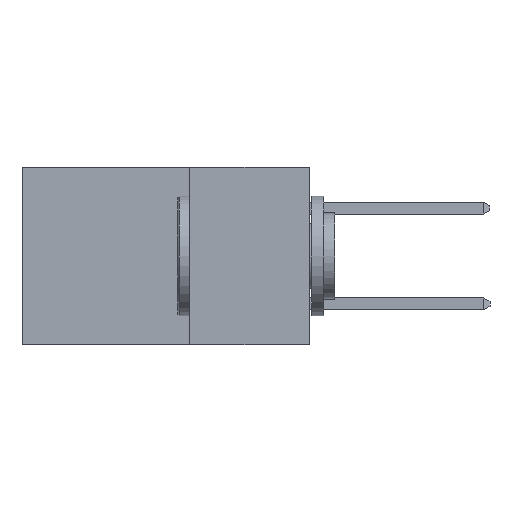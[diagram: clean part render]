
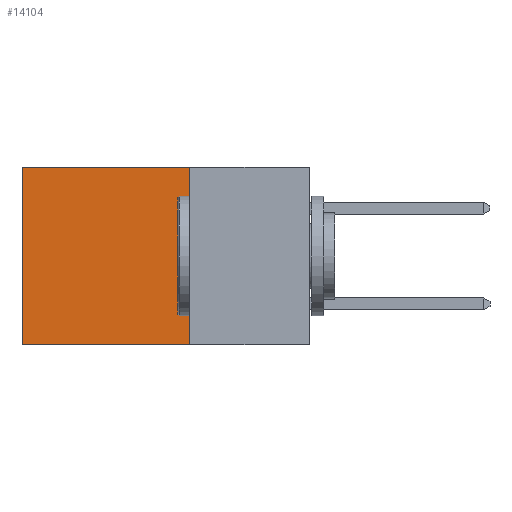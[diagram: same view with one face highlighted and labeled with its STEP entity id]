
A CAD part, left-side view. The second image highlights one B-rep face of the part: STEP entity #14104.
In plain terms, the highlighted planar face has unit normal (-1, 0, 0).
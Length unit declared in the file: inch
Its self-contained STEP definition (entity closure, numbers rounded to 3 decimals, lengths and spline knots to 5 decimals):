
#1216 = DIRECTION ( 'NONE',  ( 0., 0., -1. ) ) ;
#1329 = VERTEX_POINT ( 'NONE', #12974 ) ;
#2030 = DIRECTION ( 'NONE',  ( 0., 1., 0. ) ) ;
#2216 = CARTESIAN_POINT ( 'NONE',  ( 0.2875, 0.25, -0.37 ) ) ;
#2541 = ORIENTED_EDGE ( 'NONE', *, *, #13486, .T. ) ;
#3184 = DIRECTION ( 'NONE',  ( 1., 0., 0. ) ) ;
#3217 = DIRECTION ( 'NONE',  ( 0., 0., -1. ) ) ;
#3907 = LINE ( 'NONE', #2216, #7839 ) ;
#4141 = AXIS2_PLACEMENT_3D ( 'NONE', #9683, #3184, #4245 ) ;
#4245 = DIRECTION ( 'NONE',  ( 0., 0., -1. ) ) ;
#4846 = LINE ( 'NONE', #9719, #8121 ) ;
#5206 = CARTESIAN_POINT ( 'NONE',  ( 0.2875, 0.6, -0.37 ) ) ;
#5249 = FACE_OUTER_BOUND ( 'NONE', #9526, .T. ) ;
#5314 = DIRECTION ( 'NONE',  ( 0., 1., 0. ) ) ;
#5697 = ORIENTED_EDGE ( 'NONE', *, *, #8128, .F. ) ;
#6015 = PLANE ( 'NONE',  #4141 ) ;
#6513 = EDGE_CURVE ( 'NONE', #12170, #13741, #3907, .T. ) ;
#7839 = VECTOR ( 'NONE', #2030, 39.37008 ) ;
#7896 = CARTESIAN_POINT ( 'NONE',  ( 0.2875, 0.25, -0.37 ) ) ;
#8121 = VECTOR ( 'NONE', #3217, 39.37008 ) ;
#8128 = EDGE_CURVE ( 'NONE', #1329, #12170, #4846, .T. ) ;
#8866 = LINE ( 'NONE', #9929, #9885 ) ;
#9053 = ORIENTED_EDGE ( 'NONE', *, *, #6513, .F. ) ;
#9526 = EDGE_LOOP ( 'NONE', ( #12970, #9053, #5697, #2541 ) ) ;
#9683 = CARTESIAN_POINT ( 'NONE',  ( 0.2875, 0.25, 0. ) ) ;
#9719 = CARTESIAN_POINT ( 'NONE',  ( 0.2875, 0.25, 0. ) ) ;
#9885 = VECTOR ( 'NONE', #1216, 39.37008 ) ;
#9929 = CARTESIAN_POINT ( 'NONE',  ( 0.2875, 0.6, 0. ) ) ;
#10608 = LINE ( 'NONE', #11893, #13202 ) ;
#11893 = CARTESIAN_POINT ( 'NONE',  ( 0.2875, 0.25, 0. ) ) ;
#12129 = EDGE_CURVE ( 'NONE', #12285, #13741, #8866, .T. ) ;
#12170 = VERTEX_POINT ( 'NONE', #7896 ) ;
#12285 = VERTEX_POINT ( 'NONE', #12585 ) ;
#12585 = CARTESIAN_POINT ( 'NONE',  ( 0.2875, 0.6, 0. ) ) ;
#12970 = ORIENTED_EDGE ( 'NONE', *, *, #12129, .T. ) ;
#12974 = CARTESIAN_POINT ( 'NONE',  ( 0.2875, 0.25, 0. ) ) ;
#13202 = VECTOR ( 'NONE', #5314, 39.37008 ) ;
#13486 = EDGE_CURVE ( 'NONE', #1329, #12285, #10608, .T. ) ;
#13741 = VERTEX_POINT ( 'NONE', #5206 ) ;
#14104 = ADVANCED_FACE ( 'NONE', ( #5249 ), #6015, .F. ) ;
